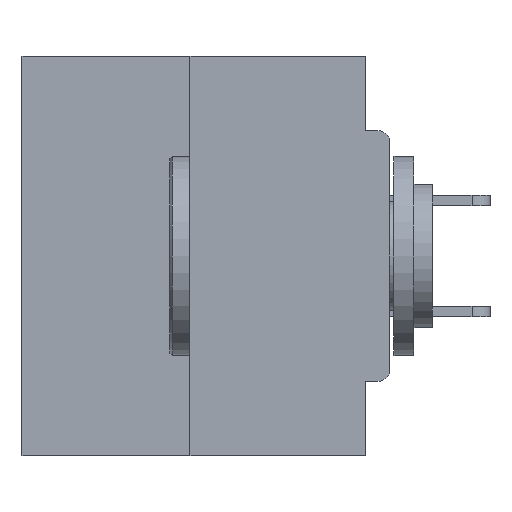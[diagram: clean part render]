
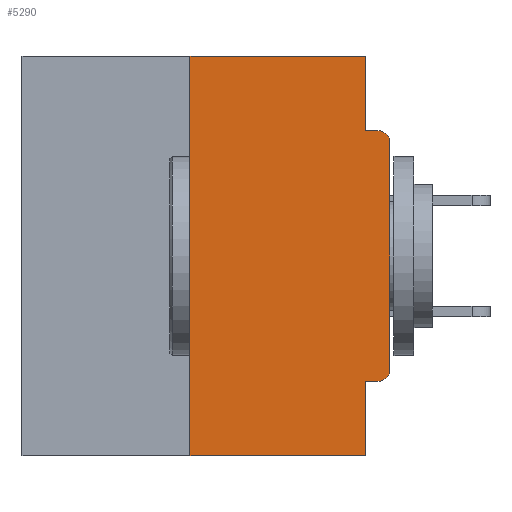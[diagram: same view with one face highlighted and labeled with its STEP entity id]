
A CAD part, left-side view. The second image highlights one B-rep face of the part: STEP entity #5290.
In plain terms, the highlighted planar face has unit normal (-1, 0, 0).
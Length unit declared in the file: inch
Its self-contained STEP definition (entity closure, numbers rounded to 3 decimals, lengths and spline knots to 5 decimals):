
#830 = AXIS2_PLACEMENT_3D ( 'NONE', #10402, #15861, #7682 ) ;
#1225 = CARTESIAN_POINT ( 'NONE',  ( 0., 0.031, 0. ) ) ;
#1236 = EDGE_LOOP ( 'NONE', ( #20383, #27707, #15608, #1693, #31805, #18006, #12975, #7482, #31999, #28324 ) ) ;
#1557 = CARTESIAN_POINT ( 'NONE',  ( 0., 0.015, -0.3915 ) ) ;
#1693 = ORIENTED_EDGE ( 'NONE', *, *, #20070, .F. ) ;
#1932 = PLANE ( 'NONE',  #5568 ) ;
#2205 = VECTOR ( 'NONE', #4843, 39.37008 ) ;
#2321 = VECTOR ( 'NONE', #31478, 39.37008 ) ;
#2516 = VERTEX_POINT ( 'NONE', #20306 ) ;
#3340 = CARTESIAN_POINT ( 'NONE',  ( 0., 0.031, 0. ) ) ;
#3586 = VERTEX_POINT ( 'NONE', #18883 ) ;
#3641 = VECTOR ( 'NONE', #19278, 39.37008 ) ;
#4132 = EDGE_CURVE ( 'NONE', #2516, #11090, #19062, .T. ) ;
#4394 = CARTESIAN_POINT ( 'NONE',  ( 0., 0., -0.0935 ) ) ;
#4794 = CARTESIAN_POINT ( 'NONE',  ( 0., 0., -0.1085 ) ) ;
#4843 = DIRECTION ( 'NONE',  ( 0., -1., 0. ) ) ;
#5143 = CARTESIAN_POINT ( 'NONE',  ( 0., 0.031, -0.5 ) ) ;
#5290 = ADVANCED_FACE ( 'NONE', ( #23166 ), #1932, .F. ) ;
#5568 = AXIS2_PLACEMENT_3D ( 'NONE', #20670, #25849, #23490 ) ;
#5839 = CARTESIAN_POINT ( 'NONE',  ( 0., 0.031, -0.4065 ) ) ;
#5849 = CARTESIAN_POINT ( 'NONE',  ( 0., 0.015, -0.0935 ) ) ;
#6630 = CARTESIAN_POINT ( 'NONE',  ( 0., 0., 0. ) ) ;
#6680 = CARTESIAN_POINT ( 'NONE',  ( 0., 0.015, -0.4065 ) ) ;
#6851 = DIRECTION ( 'NONE',  ( 0., 0., -1. ) ) ;
#7482 = ORIENTED_EDGE ( 'NONE', *, *, #28787, .T. ) ;
#7682 = DIRECTION ( 'NONE',  ( 0., 0., -1. ) ) ;
#8670 = VECTOR ( 'NONE', #30397, 39.37008 ) ;
#9817 = DIRECTION ( 'NONE',  ( 0., 0., 1. ) ) ;
#9925 = VERTEX_POINT ( 'NONE', #6680 ) ;
#10402 = CARTESIAN_POINT ( 'NONE',  ( 0., 0.015, -0.1085 ) ) ;
#10756 = VERTEX_POINT ( 'NONE', #5839 ) ;
#11090 = VERTEX_POINT ( 'NONE', #1225 ) ;
#11479 = VECTOR ( 'NONE', #9817, 39.37008 ) ;
#12726 = VERTEX_POINT ( 'NONE', #5143 ) ;
#12975 = ORIENTED_EDGE ( 'NONE', *, *, #12991, .T. ) ;
#12991 = EDGE_CURVE ( 'NONE', #21822, #14675, #18720, .T. ) ;
#14675 = VERTEX_POINT ( 'NONE', #4794 ) ;
#15140 = CARTESIAN_POINT ( 'NONE',  ( 0., 0.031, -0.5 ) ) ;
#15150 = LINE ( 'NONE', #4394, #34544 ) ;
#15244 = DIRECTION ( 'NONE',  ( 0., -1., 0. ) ) ;
#15608 = ORIENTED_EDGE ( 'NONE', *, *, #29720, .T. ) ;
#15861 = DIRECTION ( 'NONE',  ( -1., 0., 0. ) ) ;
#18006 = ORIENTED_EDGE ( 'NONE', *, *, #34332, .T. ) ;
#18345 = CARTESIAN_POINT ( 'NONE',  ( 0., 0., -0.4065 ) ) ;
#18538 = EDGE_CURVE ( 'NONE', #9925, #10756, #30104, .T. ) ;
#18624 = VECTOR ( 'NONE', #31203, 39.37008 ) ;
#18720 = LINE ( 'NONE', #6630, #11479 ) ;
#18883 = CARTESIAN_POINT ( 'NONE',  ( 0., 0.25, -0.5 ) ) ;
#19062 = LINE ( 'NONE', #22398, #18624 ) ;
#19278 = DIRECTION ( 'NONE',  ( 0., 0., -1. ) ) ;
#20070 = EDGE_CURVE ( 'NONE', #10756, #12726, #24767, .T. ) ;
#20306 = CARTESIAN_POINT ( 'NONE',  ( 0., 0.25, 0. ) ) ;
#20383 = ORIENTED_EDGE ( 'NONE', *, *, #4132, .F. ) ;
#20670 = CARTESIAN_POINT ( 'NONE',  ( 0., 0.46, 0. ) ) ;
#20756 = VERTEX_POINT ( 'NONE', #29627 ) ;
#21822 = VERTEX_POINT ( 'NONE', #24764 ) ;
#22398 = CARTESIAN_POINT ( 'NONE',  ( 0., 0.46, 0. ) ) ;
#22503 = VERTEX_POINT ( 'NONE', #5849 ) ;
#23055 = EDGE_CURVE ( 'NONE', #20756, #22503, #15150, .T. ) ;
#23166 = FACE_OUTER_BOUND ( 'NONE', #1236, .T. ) ;
#23333 = DIRECTION ( 'NONE',  ( -1., 0., 0. ) ) ;
#23490 = DIRECTION ( 'NONE',  ( 0., 0., -1. ) ) ;
#24625 = CARTESIAN_POINT ( 'NONE',  ( 0., 0.25, 0. ) ) ;
#24764 = CARTESIAN_POINT ( 'NONE',  ( 0., 0., -0.3915 ) ) ;
#24767 = LINE ( 'NONE', #15140, #30229 ) ;
#25849 = DIRECTION ( 'NONE',  ( 1., 0., 0. ) ) ;
#26202 = EDGE_CURVE ( 'NONE', #3586, #2516, #29778, .T. ) ;
#26672 = CIRCLE ( 'NONE', #830, 0.015 ) ;
#26776 = EDGE_CURVE ( 'NONE', #11090, #20756, #31011, .T. ) ;
#27707 = ORIENTED_EDGE ( 'NONE', *, *, #26202, .F. ) ;
#27933 = LINE ( 'NONE', #31803, #2205 ) ;
#28324 = ORIENTED_EDGE ( 'NONE', *, *, #26776, .F. ) ;
#28787 = EDGE_CURVE ( 'NONE', #14675, #22503, #26672, .T. ) ;
#29627 = CARTESIAN_POINT ( 'NONE',  ( 0., 0.031, -0.0935 ) ) ;
#29720 = EDGE_CURVE ( 'NONE', #3586, #12726, #27933, .T. ) ;
#29778 = LINE ( 'NONE', #24625, #8670 ) ;
#30037 = AXIS2_PLACEMENT_3D ( 'NONE', #1557, #23333, #34159 ) ;
#30104 = LINE ( 'NONE', #18345, #2321 ) ;
#30229 = VECTOR ( 'NONE', #6851, 39.37008 ) ;
#30397 = DIRECTION ( 'NONE',  ( 0., 0., 1. ) ) ;
#30799 = CIRCLE ( 'NONE', #30037, 0.015 ) ;
#31011 = LINE ( 'NONE', #3340, #3641 ) ;
#31203 = DIRECTION ( 'NONE',  ( 0., -1., 0. ) ) ;
#31478 = DIRECTION ( 'NONE',  ( 0., 1., 0. ) ) ;
#31803 = CARTESIAN_POINT ( 'NONE',  ( 0., 0.46, -0.5 ) ) ;
#31805 = ORIENTED_EDGE ( 'NONE', *, *, #18538, .F. ) ;
#31999 = ORIENTED_EDGE ( 'NONE', *, *, #23055, .F. ) ;
#34159 = DIRECTION ( 'NONE',  ( 0., 0., -1. ) ) ;
#34332 = EDGE_CURVE ( 'NONE', #9925, #21822, #30799, .T. ) ;
#34544 = VECTOR ( 'NONE', #15244, 39.37008 ) ;
